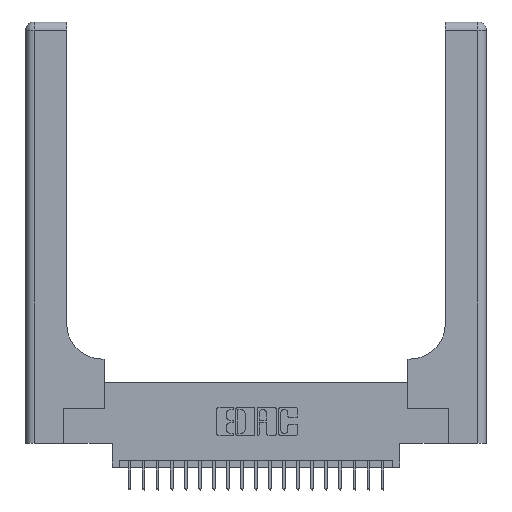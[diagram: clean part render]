
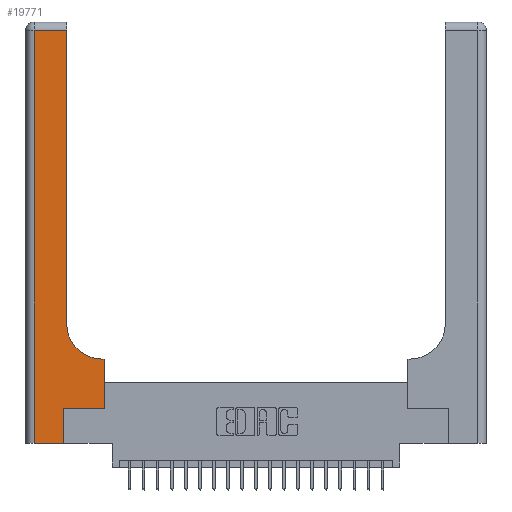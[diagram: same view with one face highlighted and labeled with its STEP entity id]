
A CAD part, top view. The second image highlights one B-rep face of the part: STEP entity #19771.
In plain terms, the highlighted planar face has unit normal (0, 0, 1).
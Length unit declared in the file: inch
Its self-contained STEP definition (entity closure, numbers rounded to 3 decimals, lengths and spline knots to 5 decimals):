
#43 = CARTESIAN_POINT ( 'NONE',  ( 0.5415, 0.6, 0.37 ) ) ;
#173 = PLANE ( 'NONE',  #15083 ) ;
#499 = EDGE_CURVE ( 'NONE', #3776, #17981, #21534, .T. ) ;
#1832 = VECTOR ( 'NONE', #8332, 39.37008 ) ;
#1838 = ORIENTED_EDGE ( 'NONE', *, *, #11203, .T. ) ;
#2006 = VERTEX_POINT ( 'NONE', #11298 ) ;
#2105 = DIRECTION ( 'NONE',  ( -1., 0., 0. ) ) ;
#2204 = LINE ( 'NONE', #2929, #16161 ) ;
#2393 = DIRECTION ( 'NONE',  ( 0., -1., 0. ) ) ;
#2609 = CIRCLE ( 'NONE', #20415, 0.25 ) ;
#2929 = CARTESIAN_POINT ( 'NONE',  ( 0.2915, 0.6, 0.37 ) ) ;
#3099 = ORIENTED_EDGE ( 'NONE', *, *, #18487, .T. ) ;
#3165 = CARTESIAN_POINT ( 'NONE',  ( 0.2915, 3., 0.37 ) ) ;
#3372 = EDGE_CURVE ( 'NONE', #15575, #20551, #4514, .T. ) ;
#3488 = ORIENTED_EDGE ( 'NONE', *, *, #5966, .T. ) ;
#3619 = EDGE_LOOP ( 'NONE', ( #3099, #18166, #1838, #14417, #3488, #20767, #18053, #17160, #19175 ) ) ;
#3776 = VERTEX_POINT ( 'NONE', #5636 ) ;
#3882 = CARTESIAN_POINT ( 'NONE',  ( 0., 3., 0.37 ) ) ;
#4514 = LINE ( 'NONE', #8404, #18392 ) ;
#4639 = CARTESIAN_POINT ( 'NONE',  ( 0.5415, 0.85, 0.37 ) ) ;
#5370 = DIRECTION ( 'NONE',  ( 0., 1., 0. ) ) ;
#5636 = CARTESIAN_POINT ( 'NONE',  ( 0.5585, 0.25, 0.37 ) ) ;
#5690 = CARTESIAN_POINT ( 'NONE',  ( 0.2915, 2.94, 0.37 ) ) ;
#5966 = EDGE_CURVE ( 'NONE', #14111, #21925, #18290, .T. ) ;
#6215 = VERTEX_POINT ( 'NONE', #43 ) ;
#6489 = DIRECTION ( 'NONE',  ( 1., 0., 0. ) ) ;
#6535 = DIRECTION ( 'NONE',  ( -1., 0., 0. ) ) ;
#6765 = LINE ( 'NONE', #19021, #1832 ) ;
#7895 = CARTESIAN_POINT ( 'NONE',  ( 0.06, 3., 0.37 ) ) ;
#8332 = DIRECTION ( 'NONE',  ( 1., 0., 0. ) ) ;
#8404 = CARTESIAN_POINT ( 'NONE',  ( 0., 2.94, 0.37 ) ) ;
#8994 = CARTESIAN_POINT ( 'NONE',  ( 0.269, 0., 0.37 ) ) ;
#9191 = FACE_OUTER_BOUND ( 'NONE', #3619, .T. ) ;
#9723 = CARTESIAN_POINT ( 'NONE',  ( 0.06, 2.94, 0.37 ) ) ;
#10279 = CARTESIAN_POINT ( 'NONE',  ( 0.2915, 0.85, 0.37 ) ) ;
#10706 = EDGE_CURVE ( 'NONE', #21925, #3776, #6765, .T. ) ;
#10813 = CARTESIAN_POINT ( 'NONE',  ( 0., 0., 0.37 ) ) ;
#11203 = EDGE_CURVE ( 'NONE', #20551, #2006, #20521, .T. ) ;
#11298 = CARTESIAN_POINT ( 'NONE',  ( 0.06, 0., 0.37 ) ) ;
#11988 = EDGE_CURVE ( 'NONE', #17981, #6215, #2204, .T. ) ;
#12462 = DIRECTION ( 'NONE',  ( 0., 1., 0. ) ) ;
#12580 = VECTOR ( 'NONE', #16191, 39.37008 ) ;
#12664 = CARTESIAN_POINT ( 'NONE',  ( 0.5585, 0.25, 0.37 ) ) ;
#13059 = DIRECTION ( 'NONE',  ( 0., 0., -1. ) ) ;
#13515 = VECTOR ( 'NONE', #19367, 39.37008 ) ;
#13957 = CARTESIAN_POINT ( 'NONE',  ( 0.269, 0., 0.37 ) ) ;
#14111 = VERTEX_POINT ( 'NONE', #8994 ) ;
#14417 = ORIENTED_EDGE ( 'NONE', *, *, #19574, .T. ) ;
#15083 = AXIS2_PLACEMENT_3D ( 'NONE', #3882, #13059, #2105 ) ;
#15263 = VERTEX_POINT ( 'NONE', #10279 ) ;
#15575 = VERTEX_POINT ( 'NONE', #5690 ) ;
#15714 = EDGE_CURVE ( 'NONE', #6215, #15263, #2609, .T. ) ;
#15778 = VECTOR ( 'NONE', #2393, 39.37008 ) ;
#16161 = VECTOR ( 'NONE', #21017, 39.37008 ) ;
#16191 = DIRECTION ( 'NONE',  ( 1., 0., 0. ) ) ;
#16830 = VECTOR ( 'NONE', #12462, 39.37008 ) ;
#17107 = VECTOR ( 'NONE', #5370, 39.37008 ) ;
#17160 = ORIENTED_EDGE ( 'NONE', *, *, #11988, .T. ) ;
#17299 = DIRECTION ( 'NONE',  ( 0., 0., -1. ) ) ;
#17328 = LINE ( 'NONE', #10813, #12580 ) ;
#17678 = LINE ( 'NONE', #3165, #17107 ) ;
#17981 = VERTEX_POINT ( 'NONE', #18675 ) ;
#18053 = ORIENTED_EDGE ( 'NONE', *, *, #499, .T. ) ;
#18166 = ORIENTED_EDGE ( 'NONE', *, *, #3372, .T. ) ;
#18290 = LINE ( 'NONE', #13957, #13515 ) ;
#18392 = VECTOR ( 'NONE', #6535, 39.37008 ) ;
#18487 = EDGE_CURVE ( 'NONE', #15263, #15575, #17678, .T. ) ;
#18675 = CARTESIAN_POINT ( 'NONE',  ( 0.5585, 0.6, 0.37 ) ) ;
#19021 = CARTESIAN_POINT ( 'NONE',  ( 0.269, 0.25, 0.37 ) ) ;
#19175 = ORIENTED_EDGE ( 'NONE', *, *, #15714, .T. ) ;
#19367 = DIRECTION ( 'NONE',  ( 0., 1., 0. ) ) ;
#19574 = EDGE_CURVE ( 'NONE', #2006, #14111, #17328, .T. ) ;
#19771 = ADVANCED_FACE ( 'NONE', ( #9191 ), #173, .F. ) ;
#19782 = CARTESIAN_POINT ( 'NONE',  ( 0.269, 0.25, 0.37 ) ) ;
#20415 = AXIS2_PLACEMENT_3D ( 'NONE', #4639, #17299, #6489 ) ;
#20521 = LINE ( 'NONE', #7895, #15778 ) ;
#20551 = VERTEX_POINT ( 'NONE', #9723 ) ;
#20767 = ORIENTED_EDGE ( 'NONE', *, *, #10706, .T. ) ;
#21017 = DIRECTION ( 'NONE',  ( -1., 0., 0. ) ) ;
#21534 = LINE ( 'NONE', #12664, #16830 ) ;
#21925 = VERTEX_POINT ( 'NONE', #19782 ) ;
